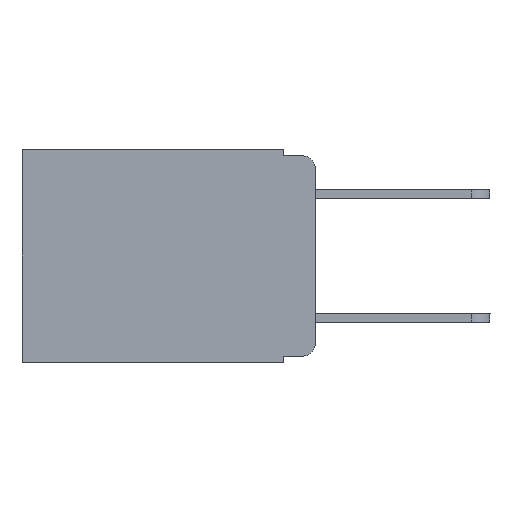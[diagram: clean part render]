
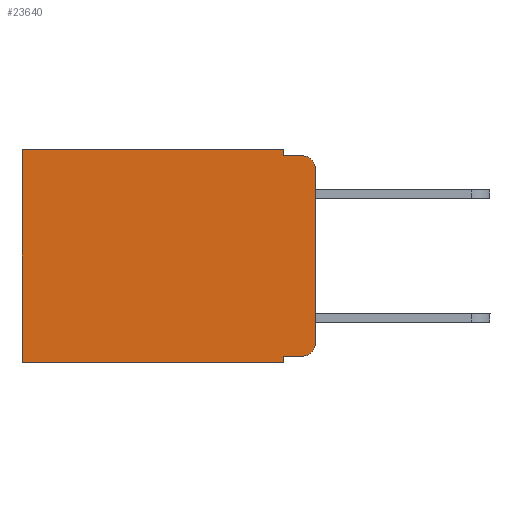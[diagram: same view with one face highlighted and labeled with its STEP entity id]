
A CAD part, left-side view. The second image highlights one B-rep face of the part: STEP entity #23640.
In plain terms, the highlighted planar face has unit normal (-1, 0, 0).
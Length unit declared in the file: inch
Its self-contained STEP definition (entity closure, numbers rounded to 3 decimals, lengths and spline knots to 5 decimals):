
#165 = EDGE_CURVE ( 'NONE', #8569, #1375, #5371, .T. ) ;
#262 = CARTESIAN_POINT ( 'NONE',  ( 0.298, 0., 0. ) ) ;
#284 = LINE ( 'NONE', #13897, #20015 ) ;
#301 = CARTESIAN_POINT ( 'NONE',  ( 0.298, 0.051, 0. ) ) ;
#864 = DIRECTION ( 'NONE',  ( 0., -1., 0. ) ) ;
#1375 = VERTEX_POINT ( 'NONE', #16128 ) ;
#2145 = LINE ( 'NONE', #2314, #23130 ) ;
#2314 = CARTESIAN_POINT ( 'NONE',  ( 0.298, 0.473, 0. ) ) ;
#2358 = DIRECTION ( 'NONE',  ( 0., -1., 0. ) ) ;
#2796 = AXIS2_PLACEMENT_3D ( 'NONE', #15044, #3570, #7241 ) ;
#3359 = CARTESIAN_POINT ( 'NONE',  ( 0.298, 0., -0.313 ) ) ;
#3570 = DIRECTION ( 'NONE',  ( -1., 0., 0. ) ) ;
#3686 = EDGE_CURVE ( 'NONE', #6778, #10032, #284, .T. ) ;
#4132 = LINE ( 'NONE', #15023, #8595 ) ;
#4432 = CARTESIAN_POINT ( 'NONE',  ( 0.298, 0.051, 0. ) ) ;
#4483 = CARTESIAN_POINT ( 'NONE',  ( 0.298, 0., -0.03 ) ) ;
#5013 = CARTESIAN_POINT ( 'NONE',  ( 0.298, 0.051, -0.343 ) ) ;
#5133 = CARTESIAN_POINT ( 'NONE',  ( 0.298, 0.051, -0.333 ) ) ;
#5371 = LINE ( 'NONE', #9628, #14697 ) ;
#6110 = CARTESIAN_POINT ( 'NONE',  ( 0.298, 0.02, -0.01 ) ) ;
#6394 = VERTEX_POINT ( 'NONE', #3359 ) ;
#6778 = VERTEX_POINT ( 'NONE', #5133 ) ;
#6896 = LINE ( 'NONE', #7256, #19216 ) ;
#6937 = ORIENTED_EDGE ( 'NONE', *, *, #19480, .T. ) ;
#7241 = DIRECTION ( 'NONE',  ( 0., 0., -1. ) ) ;
#7256 = CARTESIAN_POINT ( 'NONE',  ( 0.298, 0., 0. ) ) ;
#7413 = CARTESIAN_POINT ( 'NONE',  ( 0.298, 0.02, -0.313 ) ) ;
#7508 = AXIS2_PLACEMENT_3D ( 'NONE', #7413, #20866, #13368 ) ;
#7769 = DIRECTION ( 'NONE',  ( 0., 1., 0. ) ) ;
#7966 = PLANE ( 'NONE',  #15845 ) ;
#8017 = CARTESIAN_POINT ( 'NONE',  ( 0.298, 0.051, -0.01 ) ) ;
#8355 = EDGE_CURVE ( 'NONE', #20387, #1375, #2145, .T. ) ;
#8569 = VERTEX_POINT ( 'NONE', #5013 ) ;
#8595 = VECTOR ( 'NONE', #18965, 39.37008 ) ;
#8922 = CARTESIAN_POINT ( 'NONE',  ( 0.298, 0.02, -0.333 ) ) ;
#8970 = LINE ( 'NONE', #8017, #21892 ) ;
#9040 = VECTOR ( 'NONE', #13389, 39.37008 ) ;
#9628 = CARTESIAN_POINT ( 'NONE',  ( 0.298, 0., -0.343 ) ) ;
#9891 = DIRECTION ( 'NONE',  ( 1., 0., 0. ) ) ;
#10032 = VERTEX_POINT ( 'NONE', #8922 ) ;
#10400 = ORIENTED_EDGE ( 'NONE', *, *, #16239, .F. ) ;
#10537 = EDGE_CURVE ( 'NONE', #10868, #6394, #6896, .T. ) ;
#10868 = VERTEX_POINT ( 'NONE', #4483 ) ;
#11405 = CARTESIAN_POINT ( 'NONE',  ( 0.298, 0.051, -0.01 ) ) ;
#13368 = DIRECTION ( 'NONE',  ( 0., 0., -1. ) ) ;
#13389 = DIRECTION ( 'NONE',  ( 0., 0., -1. ) ) ;
#13600 = DIRECTION ( 'NONE',  ( 0., 1., 0. ) ) ;
#13803 = EDGE_CURVE ( 'NONE', #10032, #6394, #21968, .T. ) ;
#13834 = DIRECTION ( 'NONE',  ( 0., 0., -1. ) ) ;
#13897 = CARTESIAN_POINT ( 'NONE',  ( 0.298, 0.051, -0.333 ) ) ;
#14222 = ORIENTED_EDGE ( 'NONE', *, *, #18779, .T. ) ;
#14697 = VECTOR ( 'NONE', #7769, 39.37008 ) ;
#15023 = CARTESIAN_POINT ( 'NONE',  ( 0.298, 0.051, 0. ) ) ;
#15044 = CARTESIAN_POINT ( 'NONE',  ( 0.298, 0.02, -0.03 ) ) ;
#15084 = FACE_OUTER_BOUND ( 'NONE', #19505, .T. ) ;
#15205 = EDGE_CURVE ( 'NONE', #23509, #19900, #8970, .T. ) ;
#15845 = AXIS2_PLACEMENT_3D ( 'NONE', #21408, #9891, #13834 ) ;
#15933 = DIRECTION ( 'NONE',  ( 0., 0., -1. ) ) ;
#16128 = CARTESIAN_POINT ( 'NONE',  ( 0.298, 0.473, -0.343 ) ) ;
#16239 = EDGE_CURVE ( 'NONE', #22380, #23509, #4132, .T. ) ;
#17108 = ORIENTED_EDGE ( 'NONE', *, *, #15205, .F. ) ;
#17415 = VECTOR ( 'NONE', #13600, 39.37008 ) ;
#18621 = LINE ( 'NONE', #262, #17415 ) ;
#18779 = EDGE_CURVE ( 'NONE', #22380, #20387, #18621, .T. ) ;
#18965 = DIRECTION ( 'NONE',  ( 0., 0., -1. ) ) ;
#19216 = VECTOR ( 'NONE', #22704, 39.37008 ) ;
#19480 = EDGE_CURVE ( 'NONE', #10868, #19900, #19761, .T. ) ;
#19505 = EDGE_LOOP ( 'NONE', ( #20643, #6937, #17108, #10400, #14222, #24059, #24520, #22961, #22728, #23409 ) ) ;
#19761 = CIRCLE ( 'NONE', #2796, 0.02 ) ;
#19900 = VERTEX_POINT ( 'NONE', #6110 ) ;
#20015 = VECTOR ( 'NONE', #864, 39.37008 ) ;
#20387 = VERTEX_POINT ( 'NONE', #23750 ) ;
#20450 = LINE ( 'NONE', #301, #9040 ) ;
#20643 = ORIENTED_EDGE ( 'NONE', *, *, #10537, .F. ) ;
#20866 = DIRECTION ( 'NONE',  ( -1., 0., 0. ) ) ;
#21408 = CARTESIAN_POINT ( 'NONE',  ( 0.298, 0., 0. ) ) ;
#21892 = VECTOR ( 'NONE', #2358, 39.37008 ) ;
#21968 = CIRCLE ( 'NONE', #7508, 0.02 ) ;
#22380 = VERTEX_POINT ( 'NONE', #4432 ) ;
#22704 = DIRECTION ( 'NONE',  ( 0., 0., -1. ) ) ;
#22728 = ORIENTED_EDGE ( 'NONE', *, *, #3686, .T. ) ;
#22961 = ORIENTED_EDGE ( 'NONE', *, *, #24196, .F. ) ;
#23130 = VECTOR ( 'NONE', #15933, 39.37008 ) ;
#23409 = ORIENTED_EDGE ( 'NONE', *, *, #13803, .T. ) ;
#23509 = VERTEX_POINT ( 'NONE', #11405 ) ;
#23640 = ADVANCED_FACE ( 'NONE', ( #15084 ), #7966, .F. ) ;
#23750 = CARTESIAN_POINT ( 'NONE',  ( 0.298, 0.473, 0. ) ) ;
#24059 = ORIENTED_EDGE ( 'NONE', *, *, #8355, .T. ) ;
#24196 = EDGE_CURVE ( 'NONE', #6778, #8569, #20450, .T. ) ;
#24520 = ORIENTED_EDGE ( 'NONE', *, *, #165, .F. ) ;
